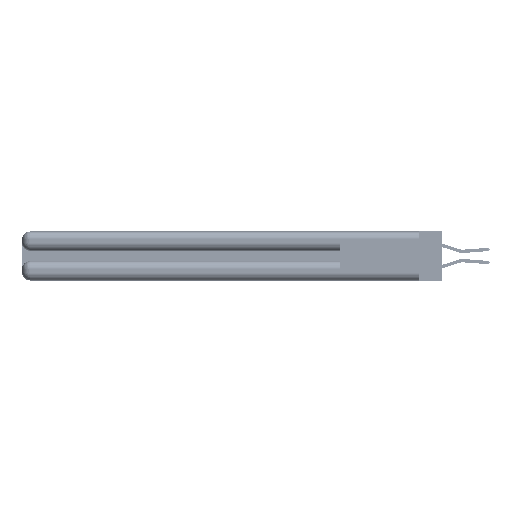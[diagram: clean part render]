
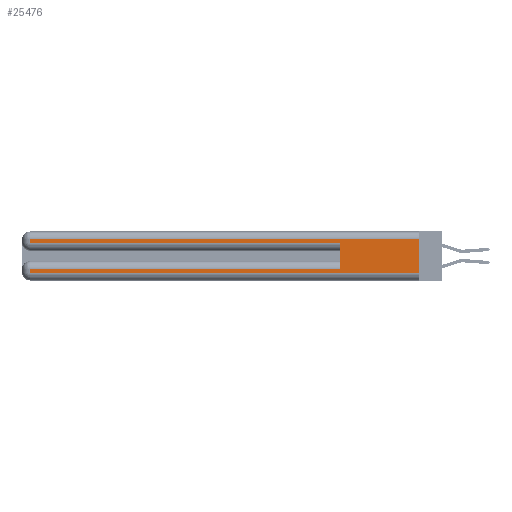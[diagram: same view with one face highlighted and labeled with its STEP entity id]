
A CAD part, left-side view. The second image highlights one B-rep face of the part: STEP entity #25476.
In plain terms, the highlighted planar face has unit normal (-1, 0, 0).
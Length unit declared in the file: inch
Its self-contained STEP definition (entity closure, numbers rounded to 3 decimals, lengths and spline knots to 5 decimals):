
#2352 = VECTOR ( 'NONE', #33069, 39.37008 ) ;
#2844 = CARTESIAN_POINT ( 'NONE',  ( 0., 0., 0.06 ) ) ;
#2942 = CARTESIAN_POINT ( 'NONE',  ( 0., 0.6, 0.285 ) ) ;
#3264 = CARTESIAN_POINT ( 'NONE',  ( 0., 2.94, 0.37 ) ) ;
#6322 = CARTESIAN_POINT ( 'NONE',  ( 0., 0.6, 0.145 ) ) ;
#7138 = LINE ( 'NONE', #15203, #51708 ) ;
#8312 = VERTEX_POINT ( 'NONE', #52674 ) ;
#8484 = VECTOR ( 'NONE', #45211, 39.37008 ) ;
#9971 = VECTOR ( 'NONE', #50860, 39.37008 ) ;
#10259 = VERTEX_POINT ( 'NONE', #36095 ) ;
#10655 = LINE ( 'NONE', #26850, #52476 ) ;
#11723 = ORIENTED_EDGE ( 'NONE', *, *, #15791, .T. ) ;
#14485 = DIRECTION ( 'NONE',  ( 1., 0., 0. ) ) ;
#15020 = CARTESIAN_POINT ( 'NONE',  ( 0., 0., 0.085 ) ) ;
#15203 = CARTESIAN_POINT ( 'NONE',  ( 0., 0., 0.37 ) ) ;
#15791 = EDGE_CURVE ( 'NONE', #8312, #37539, #44615, .T. ) ;
#16550 = EDGE_LOOP ( 'NONE', ( #27582, #53065, #35984, #16754, #34275, #50717, #43859, #11723 ) ) ;
#16754 = ORIENTED_EDGE ( 'NONE', *, *, #53726, .T. ) ;
#19148 = CARTESIAN_POINT ( 'NONE',  ( 0., 2.94, 0.085 ) ) ;
#21073 = LINE ( 'NONE', #22842, #54130 ) ;
#21358 = LINE ( 'NONE', #15020, #8484 ) ;
#21616 = VERTEX_POINT ( 'NONE', #2942 ) ;
#22842 = CARTESIAN_POINT ( 'NONE',  ( 0., 0., 0.31 ) ) ;
#23474 = VERTEX_POINT ( 'NONE', #45076 ) ;
#24413 = CARTESIAN_POINT ( 'NONE',  ( 0., 2.94, 0.37 ) ) ;
#25476 = ADVANCED_FACE ( 'NONE', ( #36114 ), #31469, .F. ) ;
#26850 = CARTESIAN_POINT ( 'NONE',  ( 0., 0., 0.285 ) ) ;
#27181 = DIRECTION ( 'NONE',  ( 0., 1., 0. ) ) ;
#27202 = EDGE_CURVE ( 'NONE', #10259, #21616, #29240, .T. ) ;
#27478 = CARTESIAN_POINT ( 'NONE',  ( 0., 2.94, 0.285 ) ) ;
#27582 = ORIENTED_EDGE ( 'NONE', *, *, #34568, .F. ) ;
#29240 = LINE ( 'NONE', #6322, #40731 ) ;
#30304 = EDGE_CURVE ( 'NONE', #41259, #8312, #32942, .T. ) ;
#31469 = PLANE ( 'NONE',  #40432 ) ;
#31653 = CARTESIAN_POINT ( 'NONE',  ( 0., 0., 0.37 ) ) ;
#31783 = VECTOR ( 'NONE', #38868, 39.37008 ) ;
#32221 = DIRECTION ( 'NONE',  ( 0., 0., 1. ) ) ;
#32631 = CARTESIAN_POINT ( 'NONE',  ( 0., 2.94, 0.31 ) ) ;
#32942 = LINE ( 'NONE', #3264, #9971 ) ;
#33069 = DIRECTION ( 'NONE',  ( 0., 0., -1. ) ) ;
#34275 = ORIENTED_EDGE ( 'NONE', *, *, #27202, .F. ) ;
#34534 = EDGE_CURVE ( 'NONE', #10259, #41259, #21358, .T. ) ;
#34568 = EDGE_CURVE ( 'NONE', #23474, #37539, #7138, .T. ) ;
#34715 = CARTESIAN_POINT ( 'NONE',  ( 0., 0., 0.06 ) ) ;
#35984 = ORIENTED_EDGE ( 'NONE', *, *, #46380, .T. ) ;
#36095 = CARTESIAN_POINT ( 'NONE',  ( 0., 0.6, 0.085 ) ) ;
#36114 = FACE_OUTER_BOUND ( 'NONE', #16550, .T. ) ;
#36873 = LINE ( 'NONE', #24413, #2352 ) ;
#37349 = VERTEX_POINT ( 'NONE', #27478 ) ;
#37539 = VERTEX_POINT ( 'NONE', #2844 ) ;
#38868 = DIRECTION ( 'NONE',  ( 0., -1., 0. ) ) ;
#40432 = AXIS2_PLACEMENT_3D ( 'NONE', #31653, #14485, #44681 ) ;
#40731 = VECTOR ( 'NONE', #32221, 39.37008 ) ;
#41073 = DIRECTION ( 'NONE',  ( 0., 0., -1. ) ) ;
#41259 = VERTEX_POINT ( 'NONE', #19148 ) ;
#41930 = EDGE_CURVE ( 'NONE', #23474, #44051, #21073, .T. ) ;
#43859 = ORIENTED_EDGE ( 'NONE', *, *, #30304, .T. ) ;
#44051 = VERTEX_POINT ( 'NONE', #32631 ) ;
#44615 = LINE ( 'NONE', #34715, #31783 ) ;
#44681 = DIRECTION ( 'NONE',  ( 0., 0., -1. ) ) ;
#45076 = CARTESIAN_POINT ( 'NONE',  ( 0., 0., 0.31 ) ) ;
#45211 = DIRECTION ( 'NONE',  ( 0., 1., 0. ) ) ;
#46380 = EDGE_CURVE ( 'NONE', #44051, #37349, #36873, .T. ) ;
#50717 = ORIENTED_EDGE ( 'NONE', *, *, #34534, .T. ) ;
#50860 = DIRECTION ( 'NONE',  ( 0., 0., -1. ) ) ;
#51708 = VECTOR ( 'NONE', #41073, 39.37008 ) ;
#52476 = VECTOR ( 'NONE', #52676, 39.37008 ) ;
#52674 = CARTESIAN_POINT ( 'NONE',  ( 0., 2.94, 0.06 ) ) ;
#52676 = DIRECTION ( 'NONE',  ( 0., -1., 0. ) ) ;
#53065 = ORIENTED_EDGE ( 'NONE', *, *, #41930, .T. ) ;
#53726 = EDGE_CURVE ( 'NONE', #37349, #21616, #10655, .T. ) ;
#54130 = VECTOR ( 'NONE', #27181, 39.37008 ) ;
